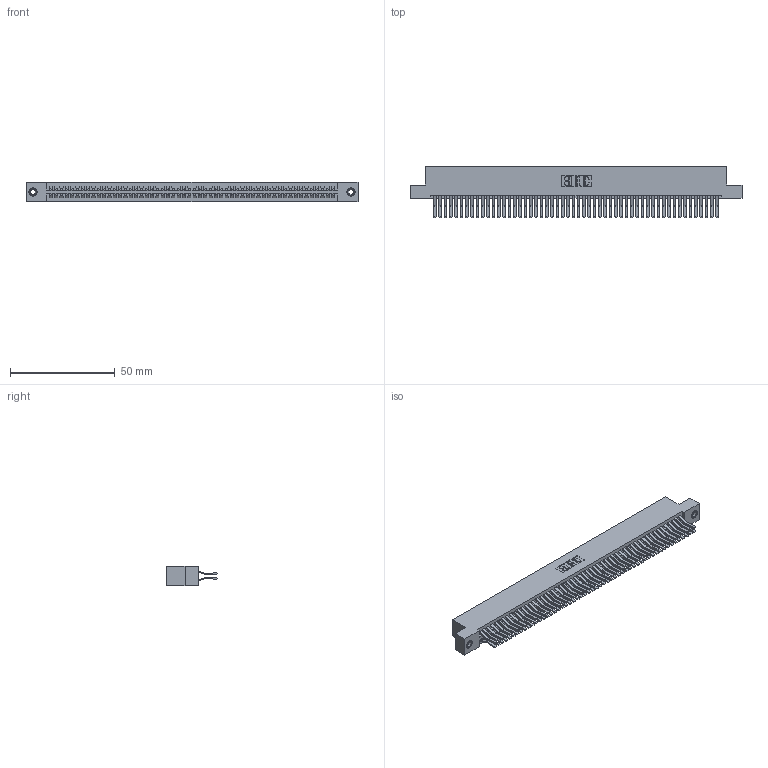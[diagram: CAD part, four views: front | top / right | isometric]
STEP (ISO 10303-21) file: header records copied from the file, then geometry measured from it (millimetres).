
FILE_DESCRIPTION (( 'STEP AP203' ), '1' );
FILE_NAME ('395-108-560-208.STEP', '2018-12-01T00:44:48', ( '' ), ( '' ), 'SwSTEP 2.0', 'SolidWorks 2016', '' );
FILE_SCHEMA (( 'CONFIG_CONTROL_DESIGN' ));
Length unit declared in the file: inch
Products named in the file (4): 395-108-560-208; 345-250-001_345-250-003-102; 345 Part_Flush Mounting Lugs - 0.156 Dia-TI; 345-292-001_560 Tail
Assembly tree (111 placements, depth 2):
  395-108-560-208
    345 Part_Flush Mounting Lugs - 0.156 Dia-TI
    345-292-001_560 Tail  x108
    345-250-001_345-250-003-102  x2
Bounding box: 158.37 x 24.45 x 9.4 mm (x, y, z)
Volume: 16196.9 mm3; surface area: 26008.2 mm2
Topology: 111 solids, 111 shells, 5802 faces, 17217 edges, 11326 vertices
Faces by surface type: plane 3676, cylinder 2110, cone 12, torus 4
Entity records: 42028 total; most frequent: CARTESIAN_POINT 7015, ORIENTED_EDGE 6942, DIRECTION 6201, EDGE_CURVE 3471, LINE 3099, VECTOR 3099, VERTEX_POINT 2308, AXIS2_PLACEMENT_3D 1551
